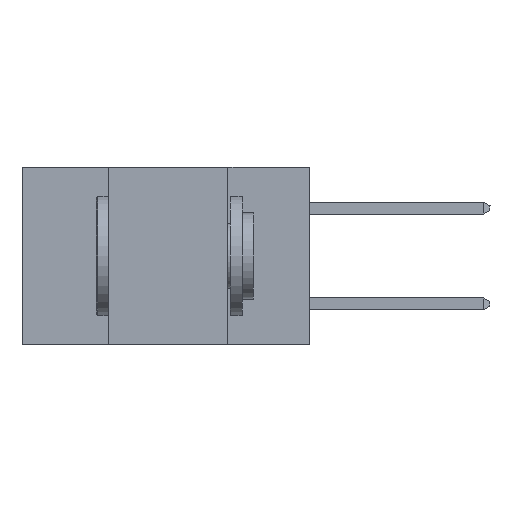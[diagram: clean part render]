
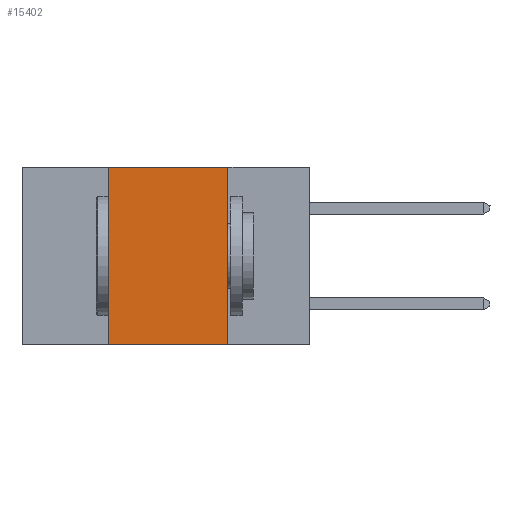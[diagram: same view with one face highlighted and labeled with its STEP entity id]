
A CAD part, left-side view. The second image highlights one B-rep face of the part: STEP entity #15402.
In plain terms, the highlighted planar face has unit normal (-1, 0, 0).
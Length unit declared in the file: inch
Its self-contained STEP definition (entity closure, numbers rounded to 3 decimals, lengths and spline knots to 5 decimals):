
#540 = VERTEX_POINT ( 'NONE', #4426 ) ;
#929 = VECTOR ( 'NONE', #5176, 39.37008 ) ;
#2053 = VERTEX_POINT ( 'NONE', #10634 ) ;
#2847 = CARTESIAN_POINT ( 'NONE',  ( 0., 0.6, -0.37 ) ) ;
#4346 = CARTESIAN_POINT ( 'NONE',  ( 0., 0.42, 0. ) ) ;
#4386 = EDGE_CURVE ( 'NONE', #2053, #540, #10594, .T. ) ;
#4426 = CARTESIAN_POINT ( 'NONE',  ( 0., 0.17, 0. ) ) ;
#4689 = EDGE_CURVE ( 'NONE', #540, #9316, #5637, .T. ) ;
#5176 = DIRECTION ( 'NONE',  ( 0., 0., -1. ) ) ;
#5258 = VECTOR ( 'NONE', #19232, 39.37008 ) ;
#5552 = PLANE ( 'NONE',  #9103 ) ;
#5637 = LINE ( 'NONE', #6987, #929 ) ;
#5849 = CARTESIAN_POINT ( 'NONE',  ( 0., 0.42, -0.37 ) ) ;
#6542 = LINE ( 'NONE', #2847, #14096 ) ;
#6987 = CARTESIAN_POINT ( 'NONE',  ( 0., 0.17, 0. ) ) ;
#7010 = CARTESIAN_POINT ( 'NONE',  ( 0., 0.6, 0. ) ) ;
#7076 = DIRECTION ( 'NONE',  ( 1., 0., 0. ) ) ;
#7201 = DIRECTION ( 'NONE',  ( 0., -1., 0. ) ) ;
#7832 = ORIENTED_EDGE ( 'NONE', *, *, #4689, .F. ) ;
#8560 = DIRECTION ( 'NONE',  ( 0., 0., -1. ) ) ;
#9103 = AXIS2_PLACEMENT_3D ( 'NONE', #7010, #7076, #8560 ) ;
#9316 = VERTEX_POINT ( 'NONE', #17146 ) ;
#9451 = EDGE_CURVE ( 'NONE', #12633, #2053, #10649, .T. ) ;
#10594 = LINE ( 'NONE', #17573, #15526 ) ;
#10634 = CARTESIAN_POINT ( 'NONE',  ( 0., 0.42, 0. ) ) ;
#10649 = LINE ( 'NONE', #4346, #5258 ) ;
#12588 = EDGE_CURVE ( 'NONE', #12633, #9316, #6542, .T. ) ;
#12633 = VERTEX_POINT ( 'NONE', #5849 ) ;
#14096 = VECTOR ( 'NONE', #17870, 39.37008 ) ;
#14398 = EDGE_LOOP ( 'NONE', ( #7832, #16304, #17124, #18512 ) ) ;
#15402 = ADVANCED_FACE ( 'NONE', ( #18425 ), #5552, .F. ) ;
#15526 = VECTOR ( 'NONE', #7201, 39.37008 ) ;
#16304 = ORIENTED_EDGE ( 'NONE', *, *, #4386, .F. ) ;
#17124 = ORIENTED_EDGE ( 'NONE', *, *, #9451, .F. ) ;
#17146 = CARTESIAN_POINT ( 'NONE',  ( 0., 0.17, -0.37 ) ) ;
#17573 = CARTESIAN_POINT ( 'NONE',  ( 0., 0.6, 0. ) ) ;
#17870 = DIRECTION ( 'NONE',  ( 0., -1., 0. ) ) ;
#18425 = FACE_OUTER_BOUND ( 'NONE', #14398, .T. ) ;
#18512 = ORIENTED_EDGE ( 'NONE', *, *, #12588, .T. ) ;
#19232 = DIRECTION ( 'NONE',  ( 0., 0., 1. ) ) ;
